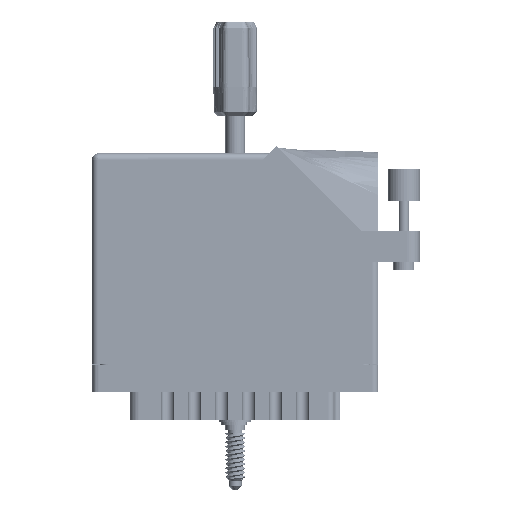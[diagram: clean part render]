
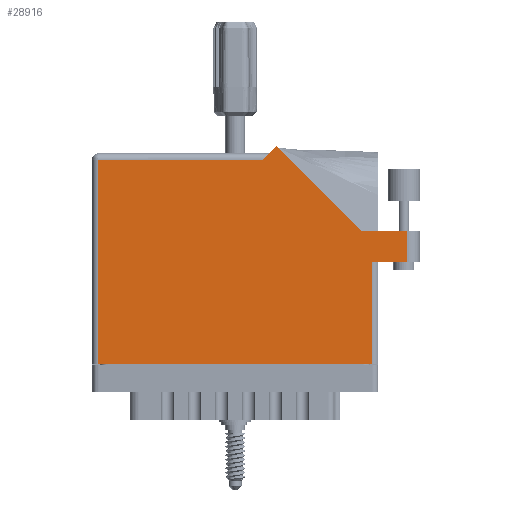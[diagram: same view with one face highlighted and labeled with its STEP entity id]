
A CAD part, front view. The second image highlights one B-rep face of the part: STEP entity #28916.
In plain terms, the highlighted face is planar.
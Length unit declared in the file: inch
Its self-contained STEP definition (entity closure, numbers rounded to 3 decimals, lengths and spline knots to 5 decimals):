
#89 = ORIENTED_EDGE ( 'NONE', *, *, #59334, .T. ) ;
#883 = CARTESIAN_POINT ( 'NONE',  ( 0., 2.03, 0. ) ) ;
#4870 = ORIENTED_EDGE ( 'NONE', *, *, #104421, .T. ) ;
#6474 = VERTEX_POINT ( 'NONE', #40885 ) ;
#7393 = VECTOR ( 'NONE', #90942, 39.37008 ) ;
#10494 = DIRECTION ( 'NONE',  ( 0., 0., -1. ) ) ;
#11772 = CARTESIAN_POINT ( 'NONE',  ( 1.77571, 2.10071, 0. ) ) ;
#11842 = EDGE_CURVE ( 'NONE', #83831, #65206, #94416, .T. ) ;
#13430 = CARTESIAN_POINT ( 'NONE',  ( 2.58942, 1.287, 0. ) ) ;
#14326 = AXIS2_PLACEMENT_3D ( 'NONE', #883, #10494, #60196 ) ;
#15073 = ORIENTED_EDGE ( 'NONE', *, *, #79283, .T. ) ;
#16647 = LINE ( 'NONE', #21617, #22010 ) ;
#18886 = VECTOR ( 'NONE', #43449, 39.37008 ) ;
#19009 = CARTESIAN_POINT ( 'NONE',  ( 0.062, 0., 0. ) ) ;
#20298 = DIRECTION ( 'NONE',  ( -0.707, 0.707, 0. ) ) ;
#21211 = EDGE_CURVE ( 'NONE', #73744, #45696, #16647, .T. ) ;
#21520 = LINE ( 'NONE', #82842, #89182 ) ;
#21556 = LINE ( 'NONE', #69457, #46827 ) ;
#21617 = CARTESIAN_POINT ( 'NONE',  ( 1.705, 2.03, 0. ) ) ;
#22010 = VECTOR ( 'NONE', #72730, 39.37008 ) ;
#26113 = VECTOR ( 'NONE', #86103, 39.37008 ) ;
#27781 = EDGE_CURVE ( 'NONE', #36025, #93180, #21556, .T. ) ;
#28916 = ADVANCED_FACE ( 'NONE', ( #45233 ), #59831, .F. ) ;
#31916 = CARTESIAN_POINT ( 'NONE',  ( 0., 1.968, 0. ) ) ;
#32726 = LINE ( 'NONE', #41449, #26113 ) ;
#33172 = VECTOR ( 'NONE', #76153, 39.37008 ) ;
#34695 = DIRECTION ( 'NONE',  ( 0., -1., 0. ) ) ;
#36025 = VERTEX_POINT ( 'NONE', #52675 ) ;
#37094 = CARTESIAN_POINT ( 'NONE',  ( 2.58942, 1.287, 0. ) ) ;
#39011 = EDGE_LOOP ( 'NONE', ( #46856, #4870, #89905, #15073, #70321, #97330, #42381, #77951, #89 ) ) ;
#40813 = EDGE_CURVE ( 'NONE', #45696, #36025, #45184, .T. ) ;
#40885 = CARTESIAN_POINT ( 'NONE',  ( 2.693, 0., 0. ) ) ;
#41449 = CARTESIAN_POINT ( 'NONE',  ( 2.755, 0.98, 0. ) ) ;
#42381 = ORIENTED_EDGE ( 'NONE', *, *, #27781, .T. ) ;
#43278 = CARTESIAN_POINT ( 'NONE',  ( 3.03, 0.98, 0. ) ) ;
#43449 = DIRECTION ( 'NONE',  ( -1., 0., 0. ) ) ;
#45184 = LINE ( 'NONE', #31916, #91362 ) ;
#45233 = FACE_OUTER_BOUND ( 'NONE', #39011, .T. ) ;
#45696 = VERTEX_POINT ( 'NONE', #50087 ) ;
#46827 = VECTOR ( 'NONE', #34695, 39.37008 ) ;
#46856 = ORIENTED_EDGE ( 'NONE', *, *, #59543, .T. ) ;
#48119 = CARTESIAN_POINT ( 'NONE',  ( 2.693, 0.98, 0. ) ) ;
#49615 = LINE ( 'NONE', #37094, #107768 ) ;
#49665 = EDGE_CURVE ( 'NONE', #93180, #6474, #21520, .T. ) ;
#50087 = CARTESIAN_POINT ( 'NONE',  ( 1.643, 1.968, 0. ) ) ;
#52675 = CARTESIAN_POINT ( 'NONE',  ( 0.062, 1.968, 0. ) ) ;
#56701 = DIRECTION ( 'NONE',  ( -1., 0., 0. ) ) ;
#59132 = CARTESIAN_POINT ( 'NONE',  ( 3.03, 1.287, 0. ) ) ;
#59334 = EDGE_CURVE ( 'NONE', #6474, #75605, #97532, .T. ) ;
#59543 = EDGE_CURVE ( 'NONE', #75605, #77644, #32726, .T. ) ;
#59831 = PLANE ( 'NONE',  #14326 ) ;
#60193 = CARTESIAN_POINT ( 'NONE',  ( 3.155, 1.287, 0. ) ) ;
#60196 = DIRECTION ( 'NONE',  ( -1., 0., 0. ) ) ;
#65206 = VERTEX_POINT ( 'NONE', #13430 ) ;
#66548 = DIRECTION ( 'NONE',  ( 1., 0., 0. ) ) ;
#69457 = CARTESIAN_POINT ( 'NONE',  ( 0.062, 0., 0. ) ) ;
#70250 = LINE ( 'NONE', #59132, #33172 ) ;
#70321 = ORIENTED_EDGE ( 'NONE', *, *, #21211, .T. ) ;
#71431 = CARTESIAN_POINT ( 'NONE',  ( 3.03, 1.287, 0. ) ) ;
#72730 = DIRECTION ( 'NONE',  ( -0.707, -0.707, 0. ) ) ;
#73744 = VERTEX_POINT ( 'NONE', #11772 ) ;
#75605 = VERTEX_POINT ( 'NONE', #86157 ) ;
#76153 = DIRECTION ( 'NONE',  ( 0., 1., 0. ) ) ;
#77644 = VERTEX_POINT ( 'NONE', #43278 ) ;
#77951 = ORIENTED_EDGE ( 'NONE', *, *, #49665, .T. ) ;
#79283 = EDGE_CURVE ( 'NONE', #65206, #73744, #49615, .T. ) ;
#82842 = CARTESIAN_POINT ( 'NONE',  ( 0., 0., 0. ) ) ;
#83831 = VERTEX_POINT ( 'NONE', #71431 ) ;
#86103 = DIRECTION ( 'NONE',  ( 1., 0., 0. ) ) ;
#86157 = CARTESIAN_POINT ( 'NONE',  ( 2.693, 0.98, 0. ) ) ;
#89182 = VECTOR ( 'NONE', #66548, 39.37008 ) ;
#89905 = ORIENTED_EDGE ( 'NONE', *, *, #11842, .T. ) ;
#90942 = DIRECTION ( 'NONE',  ( 0., 1., 0. ) ) ;
#91362 = VECTOR ( 'NONE', #56701, 39.37008 ) ;
#93180 = VERTEX_POINT ( 'NONE', #19009 ) ;
#94416 = LINE ( 'NONE', #60193, #18886 ) ;
#97330 = ORIENTED_EDGE ( 'NONE', *, *, #40813, .T. ) ;
#97532 = LINE ( 'NONE', #48119, #7393 ) ;
#104421 = EDGE_CURVE ( 'NONE', #77644, #83831, #70250, .T. ) ;
#107768 = VECTOR ( 'NONE', #20298, 39.37008 ) ;
